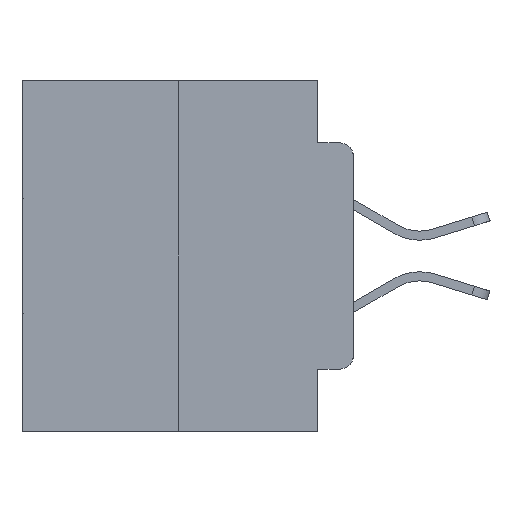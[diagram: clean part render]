
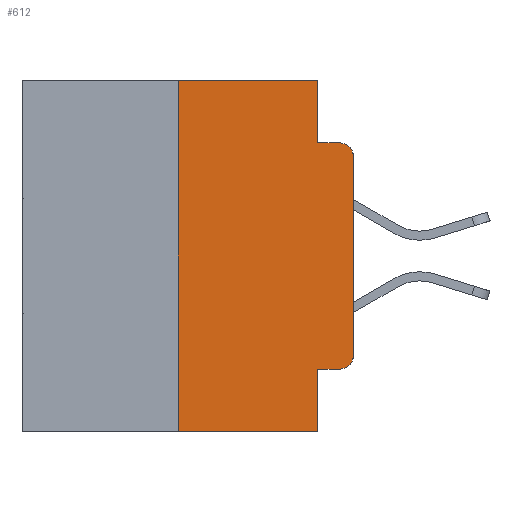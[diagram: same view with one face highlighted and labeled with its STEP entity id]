
A CAD part, left-side view. The second image highlights one B-rep face of the part: STEP entity #612.
In plain terms, the highlighted planar face has unit normal (-1, 0, 0).
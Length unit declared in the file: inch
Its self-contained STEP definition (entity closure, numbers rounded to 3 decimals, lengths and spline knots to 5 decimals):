
#46 = EDGE_CURVE ( 'NONE', #17544, #21509, #6244, .T. ) ;
#266 = LINE ( 'NONE', #5247, #11250 ) ;
#408 = CARTESIAN_POINT ( 'NONE',  ( 0., 0.25, -0.5 ) ) ;
#434 = CARTESIAN_POINT ( 'NONE',  ( 0., 0.051, 0. ) ) ;
#612 = ADVANCED_FACE ( 'NONE', ( #24706 ), #26091, .F. ) ;
#1049 = VERTEX_POINT ( 'NONE', #17170 ) ;
#1442 = DIRECTION ( 'NONE',  ( 0., -1., 0. ) ) ;
#1555 = CARTESIAN_POINT ( 'NONE',  ( 0., 0.473, 0. ) ) ;
#2004 = ORIENTED_EDGE ( 'NONE', *, *, #9529, .F. ) ;
#2165 = DIRECTION ( 'NONE',  ( -1., 0., 0. ) ) ;
#2174 = EDGE_CURVE ( 'NONE', #11315, #21509, #6028, .T. ) ;
#2296 = LINE ( 'NONE', #2983, #12616 ) ;
#2630 = DIRECTION ( 'NONE',  ( 0., 0., -1. ) ) ;
#2664 = EDGE_LOOP ( 'NONE', ( #21871, #23141, #6440, #2004, #25265, #15083, #4059, #15782, #10598, #27966 ) ) ;
#2983 = CARTESIAN_POINT ( 'NONE',  ( 0., 0., 0. ) ) ;
#3170 = DIRECTION ( 'NONE',  ( 1., 0., 0. ) ) ;
#3854 = VERTEX_POINT ( 'NONE', #25703 ) ;
#4059 = ORIENTED_EDGE ( 'NONE', *, *, #46, .T. ) ;
#4530 = VECTOR ( 'NONE', #23142, 39.37008 ) ;
#5247 = CARTESIAN_POINT ( 'NONE',  ( 0., 0.25, 0. ) ) ;
#5327 = CARTESIAN_POINT ( 'NONE',  ( 0., 0., -0.1085 ) ) ;
#6028 = LINE ( 'NONE', #13649, #27883 ) ;
#6244 = LINE ( 'NONE', #10737, #23028 ) ;
#6440 = ORIENTED_EDGE ( 'NONE', *, *, #16904, .F. ) ;
#6737 = DIRECTION ( 'NONE',  ( 0., -1., 0. ) ) ;
#7985 = DIRECTION ( 'NONE',  ( 0., 0., -1. ) ) ;
#8042 = EDGE_CURVE ( 'NONE', #17544, #24455, #266, .T. ) ;
#9529 = EDGE_CURVE ( 'NONE', #3854, #24865, #24241, .T. ) ;
#9604 = DIRECTION ( 'NONE',  ( 0., 0., 1. ) ) ;
#10598 = ORIENTED_EDGE ( 'NONE', *, *, #26162, .T. ) ;
#10737 = CARTESIAN_POINT ( 'NONE',  ( 0., 0.473, -0.5 ) ) ;
#11250 = VECTOR ( 'NONE', #25023, 39.37008 ) ;
#11315 = VERTEX_POINT ( 'NONE', #26507 ) ;
#11607 = VERTEX_POINT ( 'NONE', #20946 ) ;
#12400 = DIRECTION ( 'NONE',  ( -1., 0., 0. ) ) ;
#12616 = VECTOR ( 'NONE', #9604, 39.37008 ) ;
#12671 = VECTOR ( 'NONE', #2630, 39.37008 ) ;
#13649 = CARTESIAN_POINT ( 'NONE',  ( 0., 0.051, 0. ) ) ;
#13934 = LINE ( 'NONE', #17743, #18394 ) ;
#14201 = DIRECTION ( 'NONE',  ( 0., -1., 0. ) ) ;
#15083 = ORIENTED_EDGE ( 'NONE', *, *, #8042, .F. ) ;
#15343 = CARTESIAN_POINT ( 'NONE',  ( 0., 0.02, -0.3915 ) ) ;
#15782 = ORIENTED_EDGE ( 'NONE', *, *, #2174, .F. ) ;
#16242 = LINE ( 'NONE', #25409, #4530 ) ;
#16904 = EDGE_CURVE ( 'NONE', #24865, #11607, #13934, .T. ) ;
#17076 = EDGE_CURVE ( 'NONE', #24455, #3854, #25108, .T. ) ;
#17170 = CARTESIAN_POINT ( 'NONE',  ( 0., 0.02, -0.4115 ) ) ;
#17544 = VERTEX_POINT ( 'NONE', #408 ) ;
#17559 = DIRECTION ( 'NONE',  ( 0., 0., -1. ) ) ;
#17743 = CARTESIAN_POINT ( 'NONE',  ( 0., 0.051, -0.0885 ) ) ;
#18394 = VECTOR ( 'NONE', #6737, 39.37008 ) ;
#18413 = EDGE_CURVE ( 'NONE', #24756, #11607, #22669, .T. ) ;
#18692 = CARTESIAN_POINT ( 'NONE',  ( 0., 0.473, 0. ) ) ;
#19006 = VERTEX_POINT ( 'NONE', #23217 ) ;
#20809 = CARTESIAN_POINT ( 'NONE',  ( 0., 0.051, -0.5 ) ) ;
#20946 = CARTESIAN_POINT ( 'NONE',  ( 0., 0.02, -0.0885 ) ) ;
#21312 = AXIS2_PLACEMENT_3D ( 'NONE', #25438, #12400, #27611 ) ;
#21509 = VERTEX_POINT ( 'NONE', #20809 ) ;
#21805 = EDGE_CURVE ( 'NONE', #1049, #19006, #24923, .T. ) ;
#21871 = ORIENTED_EDGE ( 'NONE', *, *, #22723, .T. ) ;
#22465 = AXIS2_PLACEMENT_3D ( 'NONE', #15343, #2165, #17559 ) ;
#22669 = CIRCLE ( 'NONE', #21312, 0.02 ) ;
#22723 = EDGE_CURVE ( 'NONE', #19006, #24756, #2296, .T. ) ;
#23028 = VECTOR ( 'NONE', #1442, 39.37008 ) ;
#23141 = ORIENTED_EDGE ( 'NONE', *, *, #18413, .T. ) ;
#23142 = DIRECTION ( 'NONE',  ( 0., -1., 0. ) ) ;
#23204 = CARTESIAN_POINT ( 'NONE',  ( 0., 0.051, -0.0885 ) ) ;
#23217 = CARTESIAN_POINT ( 'NONE',  ( 0., 0., -0.3915 ) ) ;
#23976 = CARTESIAN_POINT ( 'NONE',  ( 0., 0.25, 0. ) ) ;
#24241 = LINE ( 'NONE', #434, #12671 ) ;
#24436 = VECTOR ( 'NONE', #14201, 39.37008 ) ;
#24455 = VERTEX_POINT ( 'NONE', #23976 ) ;
#24706 = FACE_OUTER_BOUND ( 'NONE', #2664, .T. ) ;
#24756 = VERTEX_POINT ( 'NONE', #5327 ) ;
#24865 = VERTEX_POINT ( 'NONE', #23204 ) ;
#24923 = CIRCLE ( 'NONE', #22465, 0.02 ) ;
#25023 = DIRECTION ( 'NONE',  ( 0., 0., 1. ) ) ;
#25108 = LINE ( 'NONE', #18692, #24436 ) ;
#25265 = ORIENTED_EDGE ( 'NONE', *, *, #17076, .F. ) ;
#25409 = CARTESIAN_POINT ( 'NONE',  ( 0., 0.051, -0.4115 ) ) ;
#25438 = CARTESIAN_POINT ( 'NONE',  ( 0., 0.02, -0.1085 ) ) ;
#25703 = CARTESIAN_POINT ( 'NONE',  ( 0., 0.051, 0. ) ) ;
#26091 = PLANE ( 'NONE',  #26157 ) ;
#26157 = AXIS2_PLACEMENT_3D ( 'NONE', #1555, #3170, #7985 ) ;
#26162 = EDGE_CURVE ( 'NONE', #11315, #1049, #16242, .T. ) ;
#26507 = CARTESIAN_POINT ( 'NONE',  ( 0., 0.051, -0.4115 ) ) ;
#26641 = DIRECTION ( 'NONE',  ( 0., 0., -1. ) ) ;
#27611 = DIRECTION ( 'NONE',  ( 0., 0., -1. ) ) ;
#27883 = VECTOR ( 'NONE', #26641, 39.37008 ) ;
#27966 = ORIENTED_EDGE ( 'NONE', *, *, #21805, .T. ) ;
